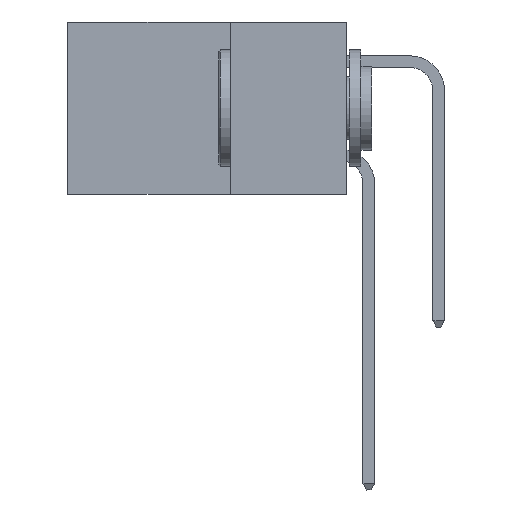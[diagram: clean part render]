
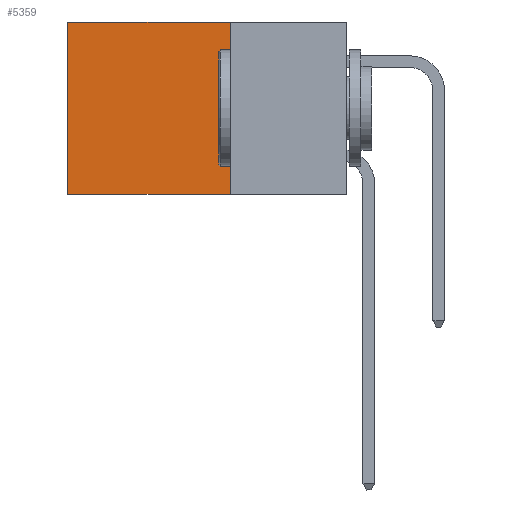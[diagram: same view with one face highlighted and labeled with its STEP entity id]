
A CAD part, left-side view. The second image highlights one B-rep face of the part: STEP entity #5359.
In plain terms, the highlighted planar face has unit normal (-1, 0, 0).
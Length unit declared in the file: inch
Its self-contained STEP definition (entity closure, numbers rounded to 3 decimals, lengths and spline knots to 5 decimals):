
#287 = LINE ( 'NONE', #5260, #7463 ) ;
#580 = CARTESIAN_POINT ( 'NONE',  ( 0.2875, 0.6, -0.37 ) ) ;
#946 = EDGE_CURVE ( 'NONE', #5901, #13440, #15668, .T. ) ;
#1314 = EDGE_LOOP ( 'NONE', ( #19437, #6834, #12356, #5763 ) ) ;
#2252 = DIRECTION ( 'NONE',  ( 0., 1., 0. ) ) ;
#2401 = CARTESIAN_POINT ( 'NONE',  ( 0.2875, 0.25, -0.37 ) ) ;
#2794 = AXIS2_PLACEMENT_3D ( 'NONE', #11305, #17425, #8342 ) ;
#4226 = CARTESIAN_POINT ( 'NONE',  ( 0.2875, 0.25, 0. ) ) ;
#4630 = DIRECTION ( 'NONE',  ( 0., 0., -1. ) ) ;
#5260 = CARTESIAN_POINT ( 'NONE',  ( 0.2875, 0.25, -0.37 ) ) ;
#5359 = ADVANCED_FACE ( 'NONE', ( #10443 ), #14420, .F. ) ;
#5763 = ORIENTED_EDGE ( 'NONE', *, *, #11738, .T. ) ;
#5901 = VERTEX_POINT ( 'NONE', #12749 ) ;
#6304 = LINE ( 'NONE', #4226, #13941 ) ;
#6834 = ORIENTED_EDGE ( 'NONE', *, *, #10085, .F. ) ;
#7463 = VECTOR ( 'NONE', #2252, 39.37008 ) ;
#7992 = CARTESIAN_POINT ( 'NONE',  ( 0.2875, 0.25, 0. ) ) ;
#8335 = CARTESIAN_POINT ( 'NONE',  ( 0.2875, 0.6, 0. ) ) ;
#8342 = DIRECTION ( 'NONE',  ( 0., 0., -1. ) ) ;
#8894 = CARTESIAN_POINT ( 'NONE',  ( 0.2875, 0.25, 0. ) ) ;
#10085 = EDGE_CURVE ( 'NONE', #11508, #13440, #287, .T. ) ;
#10443 = FACE_OUTER_BOUND ( 'NONE', #1314, .T. ) ;
#11178 = LINE ( 'NONE', #8894, #18315 ) ;
#11305 = CARTESIAN_POINT ( 'NONE',  ( 0.2875, 0.25, 0. ) ) ;
#11508 = VERTEX_POINT ( 'NONE', #2401 ) ;
#11606 = VECTOR ( 'NONE', #4630, 39.37008 ) ;
#11738 = EDGE_CURVE ( 'NONE', #11912, #5901, #11178, .T. ) ;
#11912 = VERTEX_POINT ( 'NONE', #7992 ) ;
#11914 = DIRECTION ( 'NONE',  ( 0., 1., 0. ) ) ;
#12356 = ORIENTED_EDGE ( 'NONE', *, *, #15012, .F. ) ;
#12749 = CARTESIAN_POINT ( 'NONE',  ( 0.2875, 0.6, 0. ) ) ;
#13440 = VERTEX_POINT ( 'NONE', #580 ) ;
#13941 = VECTOR ( 'NONE', #14943, 39.37008 ) ;
#14420 = PLANE ( 'NONE',  #2794 ) ;
#14943 = DIRECTION ( 'NONE',  ( 0., 0., -1. ) ) ;
#15012 = EDGE_CURVE ( 'NONE', #11912, #11508, #6304, .T. ) ;
#15668 = LINE ( 'NONE', #8335, #11606 ) ;
#17425 = DIRECTION ( 'NONE',  ( 1., 0., 0. ) ) ;
#18315 = VECTOR ( 'NONE', #11914, 39.37008 ) ;
#19437 = ORIENTED_EDGE ( 'NONE', *, *, #946, .T. ) ;
